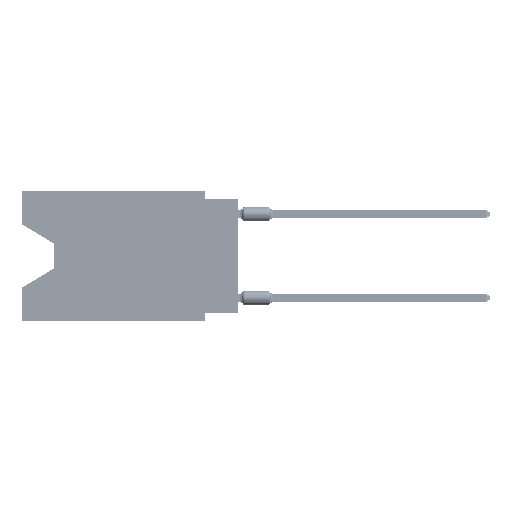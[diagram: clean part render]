
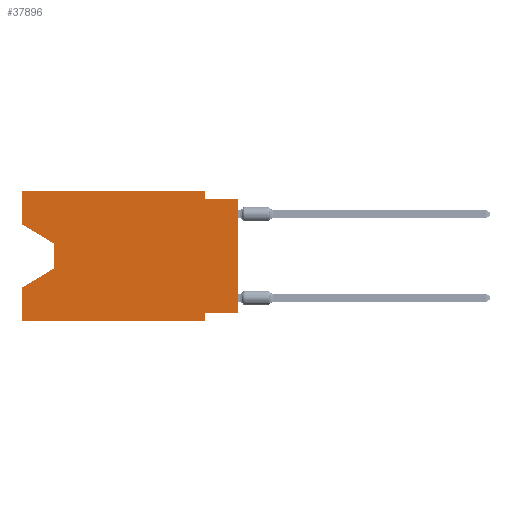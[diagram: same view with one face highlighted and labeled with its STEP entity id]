
A CAD part, left-side view. The second image highlights one B-rep face of the part: STEP entity #37896.
In plain terms, the highlighted planar face has unit normal (-1, 0, 0).
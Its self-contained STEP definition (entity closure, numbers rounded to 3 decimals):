
#1134 = CARTESIAN_POINT ( 'NONE',  ( 0., 16.383, 0. ) ) ;
#2261 = LINE ( 'NONE', #84797, #86247 ) ;
#2883 = CARTESIAN_POINT ( 'NONE',  ( 0., 13.97, -5.893 ) ) ;
#2899 = EDGE_CURVE ( 'NONE', #37645, #25779, #15883, .T. ) ;
#3149 = EDGE_CURVE ( 'NONE', #21258, #86692, #53930, .T. ) ;
#4722 = DIRECTION ( 'NONE',  ( 0., 1., 0. ) ) ;
#5672 = LINE ( 'NONE', #33036, #16824 ) ;
#7422 = ORIENTED_EDGE ( 'NONE', *, *, #82300, .T. ) ;
#9529 = DIRECTION ( 'NONE',  ( 0., 0., 1. ) ) ;
#10528 = ORIENTED_EDGE ( 'NONE', *, *, #35691, .T. ) ;
#12791 = CARTESIAN_POINT ( 'NONE',  ( 0., 16.383, 0. ) ) ;
#15738 = CARTESIAN_POINT ( 'NONE',  ( 0., 13.97, -5.893 ) ) ;
#15883 = LINE ( 'NONE', #56269, #68544 ) ;
#16824 = VECTOR ( 'NONE', #33490, 1000. ) ;
#18172 = LINE ( 'NONE', #45558, #34996 ) ;
#19167 = CARTESIAN_POINT ( 'NONE',  ( 0., 16.383, -2.546 ) ) ;
#20662 = ORIENTED_EDGE ( 'NONE', *, *, #2899, .T. ) ;
#21258 = VERTEX_POINT ( 'NONE', #40240 ) ;
#22046 = CARTESIAN_POINT ( 'NONE',  ( 0., 16.383, 0. ) ) ;
#22264 = ORIENTED_EDGE ( 'NONE', *, *, #25398, .F. ) ;
#22631 = VERTEX_POINT ( 'NONE', #56810 ) ;
#22689 = EDGE_CURVE ( 'NONE', #22631, #80018, #77441, .T. ) ;
#22842 = VERTEX_POINT ( 'NONE', #12791 ) ;
#24468 = ORIENTED_EDGE ( 'NONE', *, *, #56795, .F. ) ;
#24633 = VECTOR ( 'NONE', #76734, 1000. ) ;
#25398 = EDGE_CURVE ( 'NONE', #22842, #22631, #35254, .T. ) ;
#25779 = VERTEX_POINT ( 'NONE', #68787 ) ;
#26244 = EDGE_CURVE ( 'NONE', #68292, #43744, #75853, .T. ) ;
#28397 = VECTOR ( 'NONE', #40499, 1000. ) ;
#28942 = CARTESIAN_POINT ( 'NONE',  ( 0., 16.383, 0. ) ) ;
#30183 = VECTOR ( 'NONE', #9529, 1000. ) ;
#33036 = CARTESIAN_POINT ( 'NONE',  ( 0., 16.383, -9.906 ) ) ;
#33157 = DIRECTION ( 'NONE',  ( 0., 0., -1. ) ) ;
#33490 = DIRECTION ( 'NONE',  ( 0., -1., 0. ) ) ;
#34996 = VECTOR ( 'NONE', #4722, 1000. ) ;
#35254 = LINE ( 'NONE', #1134, #40543 ) ;
#35303 = CARTESIAN_POINT ( 'NONE',  ( 0., 0., -0.635 ) ) ;
#35691 = EDGE_CURVE ( 'NONE', #79193, #86692, #5672, .T. ) ;
#35947 = DIRECTION ( 'NONE',  ( 0., -0.855, -0.519 ) ) ;
#37645 = VERTEX_POINT ( 'NONE', #44552 ) ;
#37896 = ADVANCED_FACE ( 'NONE', ( #82612 ), #41363, .F. ) ;
#40240 = CARTESIAN_POINT ( 'NONE',  ( 0., 2.54, -9.271 ) ) ;
#40499 = DIRECTION ( 'NONE',  ( 0., 0., -1. ) ) ;
#40543 = VECTOR ( 'NONE', #41998, 1000. ) ;
#41363 = PLANE ( 'NONE',  #70079 ) ;
#41998 = DIRECTION ( 'NONE',  ( 0., -1., 0. ) ) ;
#43291 = LINE ( 'NONE', #28942, #85886 ) ;
#43744 = VERTEX_POINT ( 'NONE', #84129 ) ;
#44552 = CARTESIAN_POINT ( 'NONE',  ( 0., 0., -9.271 ) ) ;
#45558 = CARTESIAN_POINT ( 'NONE',  ( 0., 0., -9.271 ) ) ;
#46098 = VECTOR ( 'NONE', #33157, 1000. ) ;
#47501 = CARTESIAN_POINT ( 'NONE',  ( 0., 13.97, -4.013 ) ) ;
#48294 = DIRECTION ( 'NONE',  ( 0., -1., 0. ) ) ;
#49406 = DIRECTION ( 'NONE',  ( 1., 0., 0. ) ) ;
#50351 = LINE ( 'NONE', #77704, #30183 ) ;
#50782 = VECTOR ( 'NONE', #48294, 1000. ) ;
#52735 = ORIENTED_EDGE ( 'NONE', *, *, #61563, .T. ) ;
#53930 = LINE ( 'NONE', #55279, #28397 ) ;
#55279 = CARTESIAN_POINT ( 'NONE',  ( 0., 2.54, -9.906 ) ) ;
#56269 = CARTESIAN_POINT ( 'NONE',  ( 0., 0., 0. ) ) ;
#56469 = CARTESIAN_POINT ( 'NONE',  ( 0., 13.97, -4.013 ) ) ;
#56795 = EDGE_CURVE ( 'NONE', #85061, #22842, #43291, .T. ) ;
#56810 = CARTESIAN_POINT ( 'NONE',  ( 0., 2.54, 0. ) ) ;
#57411 = CARTESIAN_POINT ( 'NONE',  ( 0., 2.54, -0.635 ) ) ;
#59212 = CARTESIAN_POINT ( 'NONE',  ( 0., 2.54, -9.906 ) ) ;
#59961 = EDGE_CURVE ( 'NONE', #79193, #43744, #50351, .T. ) ;
#60067 = LINE ( 'NONE', #47501, #46098 ) ;
#61563 = EDGE_CURVE ( 'NONE', #85061, #71798, #2261, .T. ) ;
#64349 = DIRECTION ( 'NONE',  ( 0., 0., 1. ) ) ;
#64612 = VECTOR ( 'NONE', #79207, 1000. ) ;
#66072 = ORIENTED_EDGE ( 'NONE', *, *, #22689, .F. ) ;
#68292 = VERTEX_POINT ( 'NONE', #2883 ) ;
#68544 = VECTOR ( 'NONE', #71469, 1000. ) ;
#68708 = DIRECTION ( 'NONE',  ( 0., 0., -1. ) ) ;
#68787 = CARTESIAN_POINT ( 'NONE',  ( 0., 0., -0.635 ) ) ;
#70079 = AXIS2_PLACEMENT_3D ( 'NONE', #22046, #49406, #68708 ) ;
#71469 = DIRECTION ( 'NONE',  ( 0., 0., 1. ) ) ;
#71798 = VERTEX_POINT ( 'NONE', #56469 ) ;
#72498 = ORIENTED_EDGE ( 'NONE', *, *, #77239, .F. ) ;
#75853 = LINE ( 'NONE', #15738, #24633 ) ;
#76734 = DIRECTION ( 'NONE',  ( 0., 0.855, -0.519 ) ) ;
#77239 = EDGE_CURVE ( 'NONE', #37645, #21258, #18172, .T. ) ;
#77441 = LINE ( 'NONE', #85925, #64612 ) ;
#77704 = CARTESIAN_POINT ( 'NONE',  ( 0., 16.383, 0. ) ) ;
#78044 = ORIENTED_EDGE ( 'NONE', *, *, #85230, .F. ) ;
#78230 = CARTESIAN_POINT ( 'NONE',  ( 0., 16.383, -9.906 ) ) ;
#79193 = VERTEX_POINT ( 'NONE', #78230 ) ;
#79207 = DIRECTION ( 'NONE',  ( 0., 0., -1. ) ) ;
#79720 = ORIENTED_EDGE ( 'NONE', *, *, #26244, .T. ) ;
#80018 = VERTEX_POINT ( 'NONE', #57411 ) ;
#82300 = EDGE_CURVE ( 'NONE', #71798, #68292, #60067, .T. ) ;
#82612 = FACE_OUTER_BOUND ( 'NONE', #84015, .T. ) ;
#83144 = ORIENTED_EDGE ( 'NONE', *, *, #59961, .F. ) ;
#84015 = EDGE_LOOP ( 'NONE', ( #52735, #7422, #79720, #83144, #10528, #84303, #72498, #20662, #78044, #66072, #22264, #24468 ) ) ;
#84129 = CARTESIAN_POINT ( 'NONE',  ( 0., 16.383, -7.36 ) ) ;
#84303 = ORIENTED_EDGE ( 'NONE', *, *, #3149, .F. ) ;
#84797 = CARTESIAN_POINT ( 'NONE',  ( 0., 16.383, -2.546 ) ) ;
#85061 = VERTEX_POINT ( 'NONE', #19167 ) ;
#85230 = EDGE_CURVE ( 'NONE', #80018, #25779, #88652, .T. ) ;
#85886 = VECTOR ( 'NONE', #64349, 1000. ) ;
#85925 = CARTESIAN_POINT ( 'NONE',  ( 0., 2.54, 0. ) ) ;
#86247 = VECTOR ( 'NONE', #35947, 1000. ) ;
#86692 = VERTEX_POINT ( 'NONE', #59212 ) ;
#88652 = LINE ( 'NONE', #35303, #50782 ) ;
